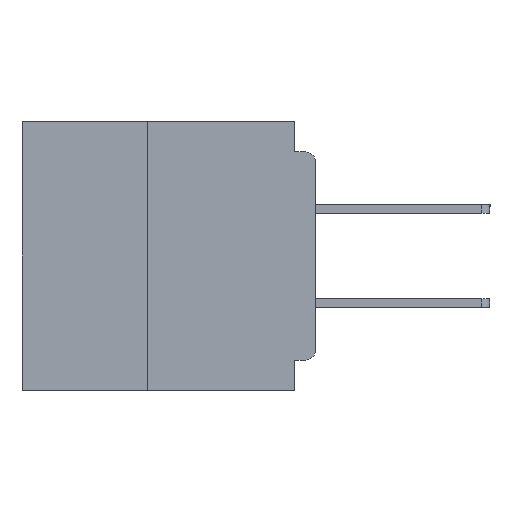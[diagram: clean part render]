
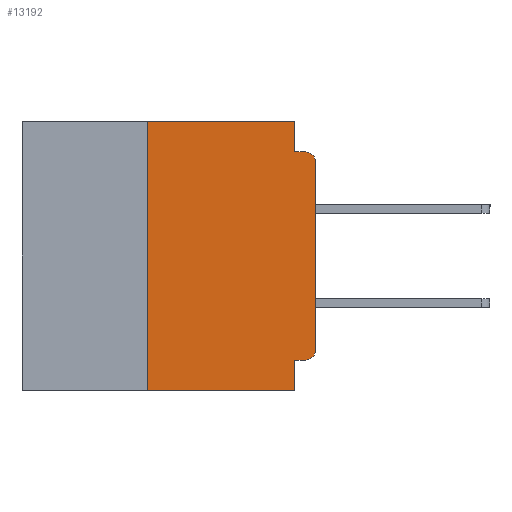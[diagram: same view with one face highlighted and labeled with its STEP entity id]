
A CAD part, left-side view. The second image highlights one B-rep face of the part: STEP entity #13192.
In plain terms, the highlighted planar face has unit normal (-1, 0, 0).
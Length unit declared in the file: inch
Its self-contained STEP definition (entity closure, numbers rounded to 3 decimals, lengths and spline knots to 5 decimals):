
#1121 = LINE ( 'NONE', #52523, #59253 ) ;
#1272 = ORIENTED_EDGE ( 'NONE', *, *, #11583, .T. ) ;
#2324 = ORIENTED_EDGE ( 'NONE', *, *, #49321, .F. ) ;
#3423 = LINE ( 'NONE', #47888, #16081 ) ;
#3641 = CARTESIAN_POINT ( 'NONE',  ( 0., 0.015, -0.06 ) ) ;
#3911 = LINE ( 'NONE', #58167, #40002 ) ;
#5173 = EDGE_CURVE ( 'NONE', #51975, #16045, #1121, .T. ) ;
#6554 = EDGE_CURVE ( 'NONE', #34922, #12036, #35650, .T. ) ;
#8441 = DIRECTION ( 'NONE',  ( 0., 0., -1. ) ) ;
#8644 = LINE ( 'NONE', #16080, #55629 ) ;
#9207 = VECTOR ( 'NONE', #30708, 39.37008 ) ;
#11489 = DIRECTION ( 'NONE',  ( 0., -1., 0. ) ) ;
#11577 = CARTESIAN_POINT ( 'NONE',  ( 0., 0.031, -0.045 ) ) ;
#11583 = EDGE_CURVE ( 'NONE', #51975, #35305, #39233, .T. ) ;
#12036 = VERTEX_POINT ( 'NONE', #14711 ) ;
#12718 = FACE_OUTER_BOUND ( 'NONE', #27831, .T. ) ;
#12909 = EDGE_CURVE ( 'NONE', #20495, #13447, #29003, .T. ) ;
#13192 = ADVANCED_FACE ( 'NONE', ( #12718 ), #29070, .F. ) ;
#13447 = VERTEX_POINT ( 'NONE', #40413 ) ;
#14122 = CARTESIAN_POINT ( 'NONE',  ( 0., 0., -0.34 ) ) ;
#14310 = VECTOR ( 'NONE', #11489, 39.37008 ) ;
#14711 = CARTESIAN_POINT ( 'NONE',  ( 0., 0.031, -0.355 ) ) ;
#16045 = VERTEX_POINT ( 'NONE', #59384 ) ;
#16080 = CARTESIAN_POINT ( 'NONE',  ( 0., 0.031, 0. ) ) ;
#16081 = VECTOR ( 'NONE', #24535, 39.37008 ) ;
#16215 = CARTESIAN_POINT ( 'NONE',  ( 0., 0.437, -0.4 ) ) ;
#18056 = CARTESIAN_POINT ( 'NONE',  ( 0., 0.015, -0.355 ) ) ;
#18850 = AXIS2_PLACEMENT_3D ( 'NONE', #54415, #26400, #59073 ) ;
#19796 = DIRECTION ( 'NONE',  ( 1., 0., 0. ) ) ;
#20084 = VERTEX_POINT ( 'NONE', #11577 ) ;
#20495 = VERTEX_POINT ( 'NONE', #33094 ) ;
#20662 = CARTESIAN_POINT ( 'NONE',  ( 0., 0.031, -0.4 ) ) ;
#22304 = ORIENTED_EDGE ( 'NONE', *, *, #5173, .F. ) ;
#23562 = EDGE_CURVE ( 'NONE', #20084, #13447, #31467, .T. ) ;
#23641 = ORIENTED_EDGE ( 'NONE', *, *, #23562, .F. ) ;
#24535 = DIRECTION ( 'NONE',  ( 0., -1., 0. ) ) ;
#25459 = DIRECTION ( 'NONE',  ( 0., 0., 1. ) ) ;
#26169 = DIRECTION ( 'NONE',  ( 0., 0., -1. ) ) ;
#26255 = AXIS2_PLACEMENT_3D ( 'NONE', #47881, #19796, #52582 ) ;
#26400 = DIRECTION ( 'NONE',  ( -1., 0., 0. ) ) ;
#26675 = ORIENTED_EDGE ( 'NONE', *, *, #12909, .T. ) ;
#27831 = EDGE_LOOP ( 'NONE', ( #31168, #26675, #23641, #49540, #44125, #22304, #1272, #2324, #35801, #41689 ) ) ;
#28576 = LINE ( 'NONE', #54193, #53469 ) ;
#29003 = CIRCLE ( 'NONE', #33675, 0.015 ) ;
#29070 = PLANE ( 'NONE',  #26255 ) ;
#29223 = DIRECTION ( 'NONE',  ( 0., 0., 1. ) ) ;
#30708 = DIRECTION ( 'NONE',  ( 0., 1., 0. ) ) ;
#31168 = ORIENTED_EDGE ( 'NONE', *, *, #56095, .T. ) ;
#31467 = LINE ( 'NONE', #60558, #42396 ) ;
#31862 = EDGE_CURVE ( 'NONE', #34922, #32768, #54197, .T. ) ;
#32768 = VERTEX_POINT ( 'NONE', #14122 ) ;
#33094 = CARTESIAN_POINT ( 'NONE',  ( 0., 0., -0.06 ) ) ;
#33675 = AXIS2_PLACEMENT_3D ( 'NONE', #3641, #36588, #8441 ) ;
#34922 = VERTEX_POINT ( 'NONE', #18056 ) ;
#35305 = VERTEX_POINT ( 'NONE', #20662 ) ;
#35650 = LINE ( 'NONE', #58680, #9207 ) ;
#35801 = ORIENTED_EDGE ( 'NONE', *, *, #6554, .F. ) ;
#36588 = DIRECTION ( 'NONE',  ( -1., 0., 0. ) ) ;
#37699 = EDGE_CURVE ( 'NONE', #16045, #43497, #3423, .T. ) ;
#37872 = EDGE_CURVE ( 'NONE', #43497, #20084, #8644, .T. ) ;
#39233 = LINE ( 'NONE', #16215, #14310 ) ;
#40002 = VECTOR ( 'NONE', #25459, 39.37008 ) ;
#40413 = CARTESIAN_POINT ( 'NONE',  ( 0., 0.015, -0.045 ) ) ;
#41689 = ORIENTED_EDGE ( 'NONE', *, *, #31862, .T. ) ;
#41946 = DIRECTION ( 'NONE',  ( 0., -1., 0. ) ) ;
#42396 = VECTOR ( 'NONE', #41946, 39.37008 ) ;
#43497 = VERTEX_POINT ( 'NONE', #55950 ) ;
#43618 = CARTESIAN_POINT ( 'NONE',  ( 0., 0.25, -0.4 ) ) ;
#44125 = ORIENTED_EDGE ( 'NONE', *, *, #37699, .F. ) ;
#47881 = CARTESIAN_POINT ( 'NONE',  ( 0., 0.437, 0. ) ) ;
#47888 = CARTESIAN_POINT ( 'NONE',  ( 0., 0.437, 0. ) ) ;
#49321 = EDGE_CURVE ( 'NONE', #12036, #35305, #28576, .T. ) ;
#49540 = ORIENTED_EDGE ( 'NONE', *, *, #37872, .F. ) ;
#51975 = VERTEX_POINT ( 'NONE', #43618 ) ;
#52523 = CARTESIAN_POINT ( 'NONE',  ( 0., 0.25, -0.4 ) ) ;
#52582 = DIRECTION ( 'NONE',  ( 0., 0., -1. ) ) ;
#53469 = VECTOR ( 'NONE', #26169, 39.37008 ) ;
#54193 = CARTESIAN_POINT ( 'NONE',  ( 0., 0.031, -0.4 ) ) ;
#54197 = CIRCLE ( 'NONE', #18850, 0.015 ) ;
#54415 = CARTESIAN_POINT ( 'NONE',  ( 0., 0.015, -0.34 ) ) ;
#55629 = VECTOR ( 'NONE', #58252, 39.37008 ) ;
#55950 = CARTESIAN_POINT ( 'NONE',  ( 0., 0.031, 0. ) ) ;
#56095 = EDGE_CURVE ( 'NONE', #32768, #20495, #3911, .T. ) ;
#58167 = CARTESIAN_POINT ( 'NONE',  ( 0., 0., 0. ) ) ;
#58252 = DIRECTION ( 'NONE',  ( 0., 0., -1. ) ) ;
#58680 = CARTESIAN_POINT ( 'NONE',  ( 0., 0., -0.355 ) ) ;
#59073 = DIRECTION ( 'NONE',  ( 0., 0., -1. ) ) ;
#59253 = VECTOR ( 'NONE', #29223, 39.37008 ) ;
#59384 = CARTESIAN_POINT ( 'NONE',  ( 0., 0.25, 0. ) ) ;
#60558 = CARTESIAN_POINT ( 'NONE',  ( 0., 0., -0.045 ) ) ;
